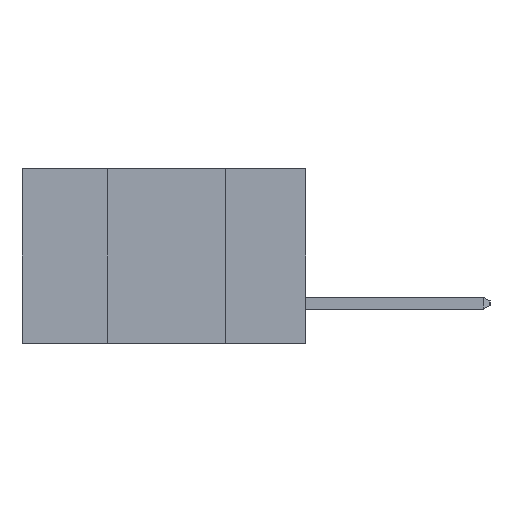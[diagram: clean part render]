
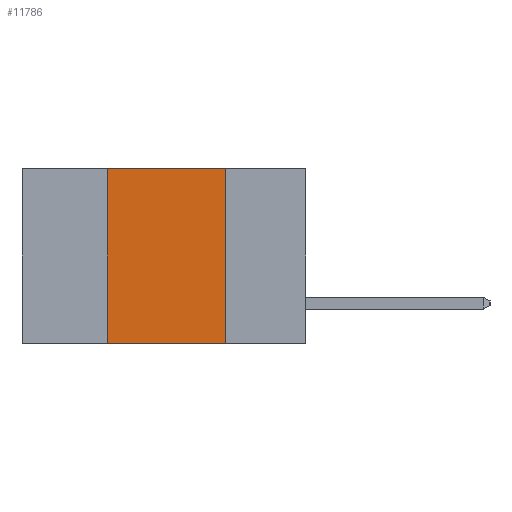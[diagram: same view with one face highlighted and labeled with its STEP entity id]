
A CAD part, left-side view. The second image highlights one B-rep face of the part: STEP entity #11786.
In plain terms, the highlighted planar face has unit normal (-1, 0, 0).
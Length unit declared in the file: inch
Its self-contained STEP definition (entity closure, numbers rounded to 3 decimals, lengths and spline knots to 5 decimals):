
#186 = CARTESIAN_POINT ( 'NONE',  ( 0., 0.17, 0. ) ) ;
#245 = CARTESIAN_POINT ( 'NONE',  ( 0., 0.6, -0.37 ) ) ;
#247 = VERTEX_POINT ( 'NONE', #3724 ) ;
#283 = AXIS2_PLACEMENT_3D ( 'NONE', #6913, #3091, #9743 ) ;
#349 = CARTESIAN_POINT ( 'NONE',  ( 0., 0.42, 0. ) ) ;
#840 = DIRECTION ( 'NONE',  ( 0., 0., -1. ) ) ;
#999 = CARTESIAN_POINT ( 'NONE',  ( 0., 0.17, -0.37 ) ) ;
#1857 = LINE ( 'NONE', #245, #11572 ) ;
#2254 = LINE ( 'NONE', #999, #7069 ) ;
#3091 = DIRECTION ( 'NONE',  ( 1., 0., 0. ) ) ;
#3394 = EDGE_CURVE ( 'NONE', #7823, #247, #1857, .T. ) ;
#3569 = ORIENTED_EDGE ( 'NONE', *, *, #8085, .F. ) ;
#3724 = CARTESIAN_POINT ( 'NONE',  ( 0., 0.17, -0.37 ) ) ;
#4188 = VERTEX_POINT ( 'NONE', #349 ) ;
#4377 = VERTEX_POINT ( 'NONE', #186 ) ;
#4675 = LINE ( 'NONE', #9784, #9438 ) ;
#5544 = ORIENTED_EDGE ( 'NONE', *, *, #9373, .F. ) ;
#6844 = EDGE_CURVE ( 'NONE', #4377, #247, #2254, .T. ) ;
#6913 = CARTESIAN_POINT ( 'NONE',  ( 0., 0.6, 0. ) ) ;
#7069 = VECTOR ( 'NONE', #840, 39.37008 ) ;
#7195 = VECTOR ( 'NONE', #11488, 39.37008 ) ;
#7324 = CARTESIAN_POINT ( 'NONE',  ( 0., 0.42, -0.37 ) ) ;
#7823 = VERTEX_POINT ( 'NONE', #7324 ) ;
#8085 = EDGE_CURVE ( 'NONE', #4188, #4377, #4675, .T. ) ;
#8347 = ORIENTED_EDGE ( 'NONE', *, *, #3394, .T. ) ;
#8799 = PLANE ( 'NONE',  #283 ) ;
#9373 = EDGE_CURVE ( 'NONE', #7823, #4188, #9699, .T. ) ;
#9438 = VECTOR ( 'NONE', #10685, 39.37008 ) ;
#9499 = FACE_OUTER_BOUND ( 'NONE', #11961, .T. ) ;
#9699 = LINE ( 'NONE', #10628, #7195 ) ;
#9743 = DIRECTION ( 'NONE',  ( 0., 0., -1. ) ) ;
#9784 = CARTESIAN_POINT ( 'NONE',  ( 0., 0.6, 0. ) ) ;
#10628 = CARTESIAN_POINT ( 'NONE',  ( 0., 0.42, -0.37 ) ) ;
#10685 = DIRECTION ( 'NONE',  ( 0., -1., 0. ) ) ;
#10790 = ORIENTED_EDGE ( 'NONE', *, *, #6844, .F. ) ;
#11488 = DIRECTION ( 'NONE',  ( 0., 0., 1. ) ) ;
#11572 = VECTOR ( 'NONE', #11623, 39.37008 ) ;
#11623 = DIRECTION ( 'NONE',  ( 0., -1., 0. ) ) ;
#11786 = ADVANCED_FACE ( 'NONE', ( #9499 ), #8799, .F. ) ;
#11961 = EDGE_LOOP ( 'NONE', ( #10790, #3569, #5544, #8347 ) ) ;
